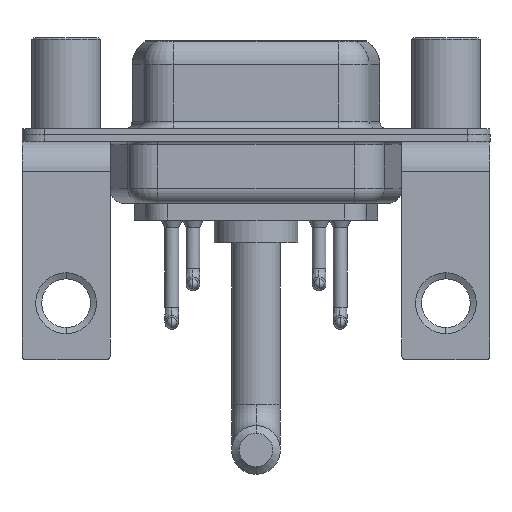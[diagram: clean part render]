
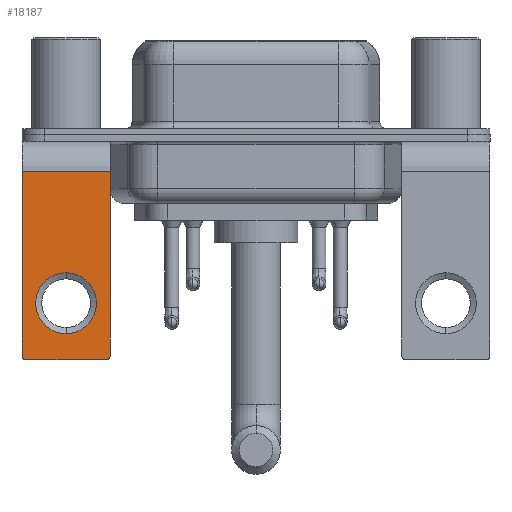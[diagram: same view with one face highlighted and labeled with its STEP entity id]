
A CAD part, front view. The second image highlights one B-rep face of the part: STEP entity #18187.
In plain terms, the highlighted planar face has unit normal (0, -1, 0).
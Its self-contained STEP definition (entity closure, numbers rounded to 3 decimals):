
#239 = DIRECTION ( 'NONE',  ( 0., -1., 0. ) ) ;
#336 = CARTESIAN_POINT ( 'NONE',  ( -2.9, -6.25, -14.55 ) ) ;
#581 = ORIENTED_EDGE ( 'NONE', *, *, #14192, .T. ) ;
#741 = LINE ( 'NONE', #1989, #11849 ) ;
#1007 = VERTEX_POINT ( 'NONE', #16056 ) ;
#1364 = DIRECTION ( 'NONE',  ( 0., 1., 0. ) ) ;
#1921 = VERTEX_POINT ( 'NONE', #5556 ) ;
#1989 = CARTESIAN_POINT ( 'NONE',  ( 2.9, -6.25, -14.8 ) ) ;
#2064 = DIRECTION ( 'NONE',  ( 0., 0., 1. ) ) ;
#2852 = AXIS2_PLACEMENT_3D ( 'NONE', #6784, #18436, #15543 ) ;
#2870 = CARTESIAN_POINT ( 'NONE',  ( 0., -6.25, -11.07 ) ) ;
#3287 = ORIENTED_EDGE ( 'NONE', *, *, #16123, .T. ) ;
#3335 = CIRCLE ( 'NONE', #16409, 2. ) ;
#3429 = VERTEX_POINT ( 'NONE', #16553 ) ;
#3827 = LINE ( 'NONE', #12750, #7056 ) ;
#4317 = DIRECTION ( 'NONE',  ( 0., 0., 1. ) ) ;
#4435 = EDGE_CURVE ( 'NONE', #3429, #15264, #13979, .T. ) ;
#4656 = CARTESIAN_POINT ( 'NONE',  ( 2.9, -6.25, -2.4 ) ) ;
#4681 = EDGE_CURVE ( 'NONE', #1007, #1921, #10918, .T. ) ;
#5556 = CARTESIAN_POINT ( 'NONE',  ( 2.9, -6.25, -14.55 ) ) ;
#5886 = ORIENTED_EDGE ( 'NONE', *, *, #4681, .T. ) ;
#6126 = VERTEX_POINT ( 'NONE', #9907 ) ;
#6132 = ORIENTED_EDGE ( 'NONE', *, *, #4435, .T. ) ;
#6408 = CIRCLE ( 'NONE', #8535, 0.25 ) ;
#6474 = EDGE_CURVE ( 'NONE', #13132, #13984, #3827, .T. ) ;
#6784 = CARTESIAN_POINT ( 'NONE',  ( 2.9, -6.25, -2.4 ) ) ;
#7056 = VECTOR ( 'NONE', #14202, 1000. ) ;
#7875 = CARTESIAN_POINT ( 'NONE',  ( -2.9, -6.25, -2.4 ) ) ;
#8117 = ORIENTED_EDGE ( 'NONE', *, *, #11228, .F. ) ;
#8203 = FACE_BOUND ( 'NONE', #17342, .T. ) ;
#8508 = ORIENTED_EDGE ( 'NONE', *, *, #8854, .T. ) ;
#8511 = DIRECTION ( 'NONE',  ( 0., 0., 1. ) ) ;
#8535 = AXIS2_PLACEMENT_3D ( 'NONE', #17290, #15852, #8511 ) ;
#8695 = VERTEX_POINT ( 'NONE', #336 ) ;
#8854 = EDGE_CURVE ( 'NONE', #13984, #8695, #16654, .T. ) ;
#9091 = AXIS2_PLACEMENT_3D ( 'NONE', #16421, #10768, #2064 ) ;
#9472 = VECTOR ( 'NONE', #18106, 1000. ) ;
#9640 = ORIENTED_EDGE ( 'NONE', *, *, #11883, .F. ) ;
#9726 = PLANE ( 'NONE',  #2852 ) ;
#9907 = CARTESIAN_POINT ( 'NONE',  ( -2.65, -6.25, -14.8 ) ) ;
#9953 = EDGE_LOOP ( 'NONE', ( #8508, #3287, #8117, #5886, #9640, #17619 ) ) ;
#10437 = DIRECTION ( 'NONE',  ( 0., 0., -1. ) ) ;
#10768 = DIRECTION ( 'NONE',  ( 0., 1., 0. ) ) ;
#10918 = CIRCLE ( 'NONE', #16735, 0.25 ) ;
#11228 = EDGE_CURVE ( 'NONE', #1007, #6126, #741, .T. ) ;
#11849 = VECTOR ( 'NONE', #13858, 1000. ) ;
#11883 = EDGE_CURVE ( 'NONE', #13132, #1921, #17716, .T. ) ;
#12563 = CARTESIAN_POINT ( 'NONE',  ( -2.9, -6.25, -2.4 ) ) ;
#12750 = CARTESIAN_POINT ( 'NONE',  ( 2.9, -6.25, -2.4 ) ) ;
#13132 = VERTEX_POINT ( 'NONE', #18275 ) ;
#13443 = CARTESIAN_POINT ( 'NONE',  ( 2.65, -6.25, -14.55 ) ) ;
#13858 = DIRECTION ( 'NONE',  ( -1., 0., 0. ) ) ;
#13979 = CIRCLE ( 'NONE', #9091, 2. ) ;
#13984 = VERTEX_POINT ( 'NONE', #12563 ) ;
#14045 = FACE_OUTER_BOUND ( 'NONE', #9953, .T. ) ;
#14192 = EDGE_CURVE ( 'NONE', #15264, #3429, #3335, .T. ) ;
#14202 = DIRECTION ( 'NONE',  ( -1., 0., 0. ) ) ;
#15264 = VERTEX_POINT ( 'NONE', #17570 ) ;
#15543 = DIRECTION ( 'NONE',  ( 0., 0., 1. ) ) ;
#15852 = DIRECTION ( 'NONE',  ( 0., -1., 0. ) ) ;
#16056 = CARTESIAN_POINT ( 'NONE',  ( 2.65, -6.25, -14.8 ) ) ;
#16123 = EDGE_CURVE ( 'NONE', #8695, #6126, #6408, .T. ) ;
#16409 = AXIS2_PLACEMENT_3D ( 'NONE', #2870, #1364, #18783 ) ;
#16421 = CARTESIAN_POINT ( 'NONE',  ( 0., -6.25, -11.07 ) ) ;
#16553 = CARTESIAN_POINT ( 'NONE',  ( 0., -6.25, -9.07 ) ) ;
#16588 = VECTOR ( 'NONE', #10437, 1000. ) ;
#16654 = LINE ( 'NONE', #7875, #9472 ) ;
#16735 = AXIS2_PLACEMENT_3D ( 'NONE', #13443, #239, #4317 ) ;
#17290 = CARTESIAN_POINT ( 'NONE',  ( -2.65, -6.25, -14.55 ) ) ;
#17342 = EDGE_LOOP ( 'NONE', ( #581, #6132 ) ) ;
#17570 = CARTESIAN_POINT ( 'NONE',  ( 0., -6.25, -13.07 ) ) ;
#17619 = ORIENTED_EDGE ( 'NONE', *, *, #6474, .T. ) ;
#17716 = LINE ( 'NONE', #4656, #16588 ) ;
#18106 = DIRECTION ( 'NONE',  ( 0., 0., -1. ) ) ;
#18187 = ADVANCED_FACE ( 'NONE', ( #8203, #14045 ), #9726, .F. ) ;
#18275 = CARTESIAN_POINT ( 'NONE',  ( 2.9, -6.25, -2.4 ) ) ;
#18436 = DIRECTION ( 'NONE',  ( 0., 1., 0. ) ) ;
#18783 = DIRECTION ( 'NONE',  ( 0., 0., 1. ) ) ;
